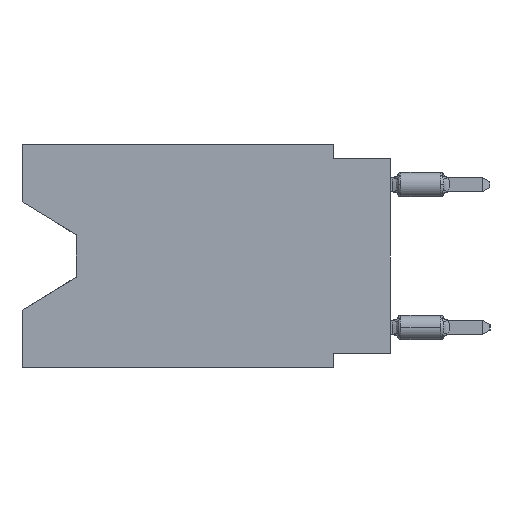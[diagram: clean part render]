
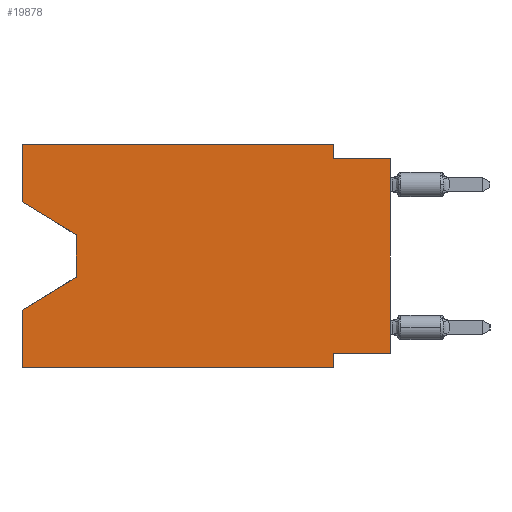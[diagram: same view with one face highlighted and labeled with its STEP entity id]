
A CAD part, left-side view. The second image highlights one B-rep face of the part: STEP entity #19878.
In plain terms, the highlighted planar face has unit normal (-1, 0, 0).
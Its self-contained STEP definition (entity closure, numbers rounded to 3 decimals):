
#38 = VERTEX_POINT ( 'NONE', #1462 ) ;
#482 = EDGE_LOOP ( 'NONE', ( #7185, #26953, #5123, #5036, #6236, #6318, #24759, #13577, #21323, #9623, #19970, #14803 ) ) ;
#653 = CARTESIAN_POINT ( 'NONE',  ( 0., 2.54, -9.906 ) ) ;
#955 = EDGE_CURVE ( 'NONE', #15565, #3777, #14307, .T. ) ;
#1091 = DIRECTION ( 'NONE',  ( 0., -0.855, -0.519 ) ) ;
#1462 = CARTESIAN_POINT ( 'NONE',  ( 0., 16.383, -9.906 ) ) ;
#1627 = DIRECTION ( 'NONE',  ( 0., 0., -1. ) ) ;
#1739 = DIRECTION ( 'NONE',  ( 0., -1., 0. ) ) ;
#2221 = CARTESIAN_POINT ( 'NONE',  ( 0., 2.54, 0. ) ) ;
#2266 = EDGE_CURVE ( 'NONE', #38, #11127, #16928, .T. ) ;
#2850 = LINE ( 'NONE', #25682, #9587 ) ;
#3196 = EDGE_CURVE ( 'NONE', #27082, #22668, #25551, .T. ) ;
#3205 = EDGE_CURVE ( 'NONE', #15833, #14969, #2850, .T. ) ;
#3378 = EDGE_CURVE ( 'NONE', #18877, #27082, #27170, .T. ) ;
#3777 = VERTEX_POINT ( 'NONE', #5679 ) ;
#4148 = LINE ( 'NONE', #25489, #13905 ) ;
#5036 = ORIENTED_EDGE ( 'NONE', *, *, #2266, .F. ) ;
#5123 = ORIENTED_EDGE ( 'NONE', *, *, #25278, .T. ) ;
#5370 = EDGE_CURVE ( 'NONE', #15982, #15565, #8103, .T. ) ;
#5679 = CARTESIAN_POINT ( 'NONE',  ( 0., 0., -0.635 ) ) ;
#5708 = CARTESIAN_POINT ( 'NONE',  ( 0., 0., -9.271 ) ) ;
#6236 = ORIENTED_EDGE ( 'NONE', *, *, #13254, .T. ) ;
#6318 = ORIENTED_EDGE ( 'NONE', *, *, #3196, .F. ) ;
#6592 = DIRECTION ( 'NONE',  ( 0., 0., 1. ) ) ;
#7185 = ORIENTED_EDGE ( 'NONE', *, *, #19028, .T. ) ;
#7364 = VECTOR ( 'NONE', #6592, 1000. ) ;
#7556 = DIRECTION ( 'NONE',  ( 0., 0.855, -0.519 ) ) ;
#7708 = CARTESIAN_POINT ( 'NONE',  ( 0., 0., -0.635 ) ) ;
#7838 = VECTOR ( 'NONE', #9000, 1000. ) ;
#7965 = DIRECTION ( 'NONE',  ( 0., 0., -1. ) ) ;
#8030 = CARTESIAN_POINT ( 'NONE',  ( 0., 16.383, 0. ) ) ;
#8103 = LINE ( 'NONE', #22335, #9100 ) ;
#8445 = EDGE_CURVE ( 'NONE', #10921, #22419, #9841, .T. ) ;
#8907 = CARTESIAN_POINT ( 'NONE',  ( 0., 16.383, 0. ) ) ;
#9000 = DIRECTION ( 'NONE',  ( 0., 0., -1. ) ) ;
#9034 = CARTESIAN_POINT ( 'NONE',  ( 0., 13.97, -4.013 ) ) ;
#9100 = VECTOR ( 'NONE', #26582, 1000. ) ;
#9489 = DIRECTION ( 'NONE',  ( 0., 0., 1. ) ) ;
#9587 = VECTOR ( 'NONE', #17303, 1000. ) ;
#9623 = ORIENTED_EDGE ( 'NONE', *, *, #5370, .F. ) ;
#9841 = LINE ( 'NONE', #16071, #16250 ) ;
#10921 = VERTEX_POINT ( 'NONE', #9034 ) ;
#11127 = VERTEX_POINT ( 'NONE', #15071 ) ;
#11420 = EDGE_CURVE ( 'NONE', #14969, #15982, #26638, .T. ) ;
#11502 = LINE ( 'NONE', #19931, #22089 ) ;
#12205 = FACE_OUTER_BOUND ( 'NONE', #482, .T. ) ;
#12461 = CARTESIAN_POINT ( 'NONE',  ( 0., 16.383, 0. ) ) ;
#12511 = VECTOR ( 'NONE', #7556, 1000. ) ;
#13005 = CARTESIAN_POINT ( 'NONE',  ( 0., 0., -9.271 ) ) ;
#13254 = EDGE_CURVE ( 'NONE', #38, #22668, #4148, .T. ) ;
#13577 = ORIENTED_EDGE ( 'NONE', *, *, #13604, .T. ) ;
#13604 = EDGE_CURVE ( 'NONE', #18877, #3777, #22333, .T. ) ;
#13905 = VECTOR ( 'NONE', #21088, 1000. ) ;
#14307 = LINE ( 'NONE', #7708, #25802 ) ;
#14803 = ORIENTED_EDGE ( 'NONE', *, *, #3205, .F. ) ;
#14969 = VERTEX_POINT ( 'NONE', #20458 ) ;
#15071 = CARTESIAN_POINT ( 'NONE',  ( 0., 16.383, -7.36 ) ) ;
#15393 = CARTESIAN_POINT ( 'NONE',  ( 0., 2.54, -9.906 ) ) ;
#15565 = VERTEX_POINT ( 'NONE', #21646 ) ;
#15833 = VERTEX_POINT ( 'NONE', #24526 ) ;
#15982 = VERTEX_POINT ( 'NONE', #2221 ) ;
#16071 = CARTESIAN_POINT ( 'NONE',  ( 0., 13.97, -4.013 ) ) ;
#16250 = VECTOR ( 'NONE', #1627, 1000. ) ;
#16261 = CARTESIAN_POINT ( 'NONE',  ( 0., 0., 0. ) ) ;
#16928 = LINE ( 'NONE', #8907, #7364 ) ;
#17303 = DIRECTION ( 'NONE',  ( 0., 0., 1. ) ) ;
#18188 = CARTESIAN_POINT ( 'NONE',  ( 0., 13.97, -5.893 ) ) ;
#18717 = DIRECTION ( 'NONE',  ( 0., -1., 0. ) ) ;
#18844 = VECTOR ( 'NONE', #20449, 1000. ) ;
#18877 = VERTEX_POINT ( 'NONE', #13005 ) ;
#19028 = EDGE_CURVE ( 'NONE', #15833, #10921, #11502, .T. ) ;
#19878 = ADVANCED_FACE ( 'NONE', ( #12205 ), #21038, .F. ) ;
#19931 = CARTESIAN_POINT ( 'NONE',  ( 0., 16.383, -2.546 ) ) ;
#19970 = ORIENTED_EDGE ( 'NONE', *, *, #11420, .F. ) ;
#20089 = LINE ( 'NONE', #26422, #12511 ) ;
#20449 = DIRECTION ( 'NONE',  ( 0., 1., 0. ) ) ;
#20458 = CARTESIAN_POINT ( 'NONE',  ( 0., 16.383, 0. ) ) ;
#20642 = DIRECTION ( 'NONE',  ( 1., 0., 0. ) ) ;
#21038 = PLANE ( 'NONE',  #27066 ) ;
#21088 = DIRECTION ( 'NONE',  ( 0., -1., 0. ) ) ;
#21323 = ORIENTED_EDGE ( 'NONE', *, *, #955, .F. ) ;
#21646 = CARTESIAN_POINT ( 'NONE',  ( 0., 2.54, -0.635 ) ) ;
#22089 = VECTOR ( 'NONE', #1091, 1000. ) ;
#22333 = LINE ( 'NONE', #16261, #25067 ) ;
#22335 = CARTESIAN_POINT ( 'NONE',  ( 0., 2.54, 0. ) ) ;
#22419 = VERTEX_POINT ( 'NONE', #18188 ) ;
#22635 = VECTOR ( 'NONE', #1739, 1000. ) ;
#22668 = VERTEX_POINT ( 'NONE', #15393 ) ;
#24351 = CARTESIAN_POINT ( 'NONE',  ( 0., 2.54, -9.271 ) ) ;
#24526 = CARTESIAN_POINT ( 'NONE',  ( 0., 16.383, -2.546 ) ) ;
#24759 = ORIENTED_EDGE ( 'NONE', *, *, #3378, .F. ) ;
#25067 = VECTOR ( 'NONE', #9489, 1000. ) ;
#25278 = EDGE_CURVE ( 'NONE', #22419, #11127, #20089, .T. ) ;
#25489 = CARTESIAN_POINT ( 'NONE',  ( 0., 16.383, -9.906 ) ) ;
#25551 = LINE ( 'NONE', #653, #7838 ) ;
#25682 = CARTESIAN_POINT ( 'NONE',  ( 0., 16.383, 0. ) ) ;
#25802 = VECTOR ( 'NONE', #18717, 1000. ) ;
#26422 = CARTESIAN_POINT ( 'NONE',  ( 0., 13.97, -5.893 ) ) ;
#26582 = DIRECTION ( 'NONE',  ( 0., 0., -1. ) ) ;
#26638 = LINE ( 'NONE', #8030, #22635 ) ;
#26953 = ORIENTED_EDGE ( 'NONE', *, *, #8445, .T. ) ;
#27066 = AXIS2_PLACEMENT_3D ( 'NONE', #12461, #20642, #7965 ) ;
#27082 = VERTEX_POINT ( 'NONE', #24351 ) ;
#27170 = LINE ( 'NONE', #5708, #18844 ) ;
